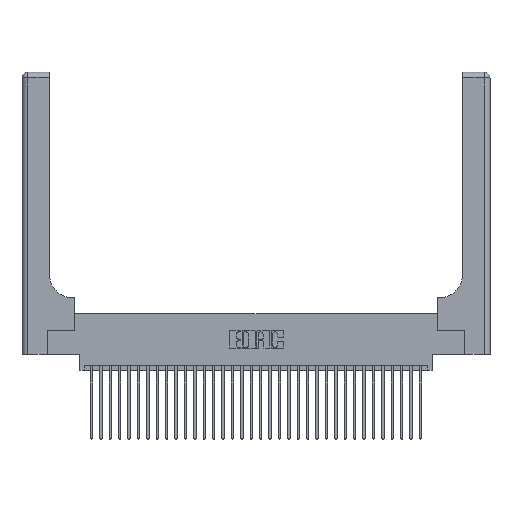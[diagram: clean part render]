
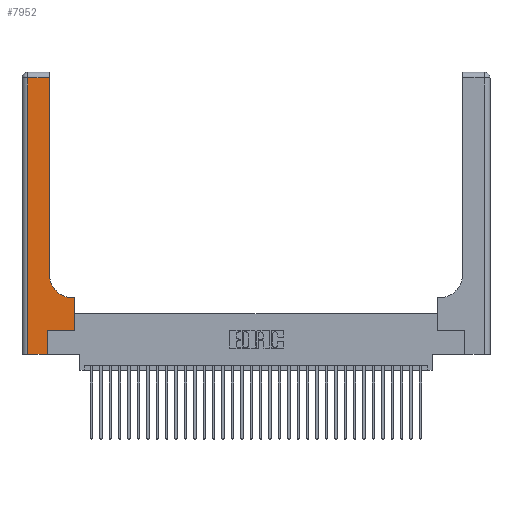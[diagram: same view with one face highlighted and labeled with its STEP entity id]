
A CAD part, top view. The second image highlights one B-rep face of the part: STEP entity #7952.
In plain terms, the highlighted planar face has unit normal (0, 0, 1).
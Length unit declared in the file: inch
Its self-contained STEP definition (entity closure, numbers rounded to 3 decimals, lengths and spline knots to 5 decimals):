
#53 = ORIENTED_EDGE ( 'NONE', *, *, #33760, .T. ) ;
#220 = ORIENTED_EDGE ( 'NONE', *, *, #10507, .T. ) ;
#1835 = CARTESIAN_POINT ( 'NONE',  ( 0.269, 0.25, 0.37 ) ) ;
#1864 = VERTEX_POINT ( 'NONE', #5188 ) ;
#2416 = CARTESIAN_POINT ( 'NONE',  ( 0.06, 2.94, 0.37 ) ) ;
#2427 = ORIENTED_EDGE ( 'NONE', *, *, #21589, .T. ) ;
#2429 = CARTESIAN_POINT ( 'NONE',  ( 0., 3., 0.37 ) ) ;
#2832 = AXIS2_PLACEMENT_3D ( 'NONE', #3322, #21878, #16112 ) ;
#3148 = EDGE_CURVE ( 'NONE', #29136, #28993, #34333, .T. ) ;
#3322 = CARTESIAN_POINT ( 'NONE',  ( 0.5415, 0.85, 0.37 ) ) ;
#3689 = DIRECTION ( 'NONE',  ( 0., 1., 0. ) ) ;
#4257 = VERTEX_POINT ( 'NONE', #28048 ) ;
#5188 = CARTESIAN_POINT ( 'NONE',  ( 0.2915, 2.94, 0.37 ) ) ;
#6335 = LINE ( 'NONE', #16570, #33806 ) ;
#6635 = VECTOR ( 'NONE', #23419, 39.37008 ) ;
#7905 = CARTESIAN_POINT ( 'NONE',  ( 0.2915, 3., 0.37 ) ) ;
#7952 = ADVANCED_FACE ( 'NONE', ( #21160 ), #18320, .F. ) ;
#8855 = CARTESIAN_POINT ( 'NONE',  ( 0.5585, 0.25, 0.37 ) ) ;
#9536 = EDGE_CURVE ( 'NONE', #32376, #24922, #28514, .T. ) ;
#10067 = ORIENTED_EDGE ( 'NONE', *, *, #9536, .T. ) ;
#10507 = EDGE_CURVE ( 'NONE', #24922, #33377, #11830, .T. ) ;
#10815 = EDGE_LOOP ( 'NONE', ( #32452, #2427, #19612, #15240, #53, #33770, #24573, #10067, #220 ) ) ;
#11830 = CIRCLE ( 'NONE', #2832, 0.25 ) ;
#12176 = VECTOR ( 'NONE', #25316, 39.37008 ) ;
#12636 = DIRECTION ( 'NONE',  ( 1., 0., 0. ) ) ;
#12757 = VECTOR ( 'NONE', #30065, 39.37008 ) ;
#13221 = VECTOR ( 'NONE', #3689, 39.37008 ) ;
#13492 = LINE ( 'NONE', #1835, #16812 ) ;
#13752 = LINE ( 'NONE', #7905, #24972 ) ;
#13782 = CARTESIAN_POINT ( 'NONE',  ( 0.5585, 0.25, 0.37 ) ) ;
#14566 = LINE ( 'NONE', #18322, #6635 ) ;
#15240 = ORIENTED_EDGE ( 'NONE', *, *, #3148, .T. ) ;
#16108 = DIRECTION ( 'NONE',  ( -1., 0., 0. ) ) ;
#16112 = DIRECTION ( 'NONE',  ( 1., 0., 0. ) ) ;
#16570 = CARTESIAN_POINT ( 'NONE',  ( 0., 2.94, 0.37 ) ) ;
#16812 = VECTOR ( 'NONE', #12636, 39.37008 ) ;
#18320 = PLANE ( 'NONE',  #21254 ) ;
#18322 = CARTESIAN_POINT ( 'NONE',  ( 0.06, 3., 0.37 ) ) ;
#19193 = LINE ( 'NONE', #28199, #12176 ) ;
#19612 = ORIENTED_EDGE ( 'NONE', *, *, #23585, .T. ) ;
#20281 = LINE ( 'NONE', #8855, #13221 ) ;
#20591 = DIRECTION ( 'NONE',  ( 1., 0., 0. ) ) ;
#21160 = FACE_OUTER_BOUND ( 'NONE', #10815, .T. ) ;
#21254 = AXIS2_PLACEMENT_3D ( 'NONE', #2429, #31688, #16108 ) ;
#21398 = VERTEX_POINT ( 'NONE', #2416 ) ;
#21589 = EDGE_CURVE ( 'NONE', #1864, #21398, #6335, .T. ) ;
#21878 = DIRECTION ( 'NONE',  ( 0., 0., -1. ) ) ;
#23419 = DIRECTION ( 'NONE',  ( 0., -1., 0. ) ) ;
#23510 = DIRECTION ( 'NONE',  ( 0., 1., 0. ) ) ;
#23585 = EDGE_CURVE ( 'NONE', #21398, #29136, #14566, .T. ) ;
#24202 = CARTESIAN_POINT ( 'NONE',  ( 0.5415, 0.6, 0.37 ) ) ;
#24230 = CARTESIAN_POINT ( 'NONE',  ( 0.269, 0., 0.37 ) ) ;
#24573 = ORIENTED_EDGE ( 'NONE', *, *, #31094, .T. ) ;
#24921 = DIRECTION ( 'NONE',  ( -1., 0., 0. ) ) ;
#24922 = VERTEX_POINT ( 'NONE', #24202 ) ;
#24972 = VECTOR ( 'NONE', #23510, 39.37008 ) ;
#25316 = DIRECTION ( 'NONE',  ( 0., 1., 0. ) ) ;
#28048 = CARTESIAN_POINT ( 'NONE',  ( 0.269, 0.25, 0.37 ) ) ;
#28199 = CARTESIAN_POINT ( 'NONE',  ( 0.269, 0., 0.37 ) ) ;
#28514 = LINE ( 'NONE', #32996, #12757 ) ;
#28728 = CARTESIAN_POINT ( 'NONE',  ( 0.5585, 0.6, 0.37 ) ) ;
#28903 = CARTESIAN_POINT ( 'NONE',  ( 0., 0., 0.37 ) ) ;
#28993 = VERTEX_POINT ( 'NONE', #24230 ) ;
#29136 = VERTEX_POINT ( 'NONE', #32922 ) ;
#30065 = DIRECTION ( 'NONE',  ( -1., 0., 0. ) ) ;
#30992 = VERTEX_POINT ( 'NONE', #13782 ) ;
#31094 = EDGE_CURVE ( 'NONE', #30992, #32376, #20281, .T. ) ;
#31688 = DIRECTION ( 'NONE',  ( 0., 0., -1. ) ) ;
#31953 = CARTESIAN_POINT ( 'NONE',  ( 0.2915, 0.85, 0.37 ) ) ;
#32376 = VERTEX_POINT ( 'NONE', #28728 ) ;
#32452 = ORIENTED_EDGE ( 'NONE', *, *, #34387, .T. ) ;
#32465 = EDGE_CURVE ( 'NONE', #4257, #30992, #13492, .T. ) ;
#32639 = VECTOR ( 'NONE', #20591, 39.37008 ) ;
#32922 = CARTESIAN_POINT ( 'NONE',  ( 0.06, 0., 0.37 ) ) ;
#32996 = CARTESIAN_POINT ( 'NONE',  ( 0.2915, 0.6, 0.37 ) ) ;
#33377 = VERTEX_POINT ( 'NONE', #31953 ) ;
#33760 = EDGE_CURVE ( 'NONE', #28993, #4257, #19193, .T. ) ;
#33770 = ORIENTED_EDGE ( 'NONE', *, *, #32465, .T. ) ;
#33806 = VECTOR ( 'NONE', #24921, 39.37008 ) ;
#34333 = LINE ( 'NONE', #28903, #32639 ) ;
#34387 = EDGE_CURVE ( 'NONE', #33377, #1864, #13752, .T. ) ;
